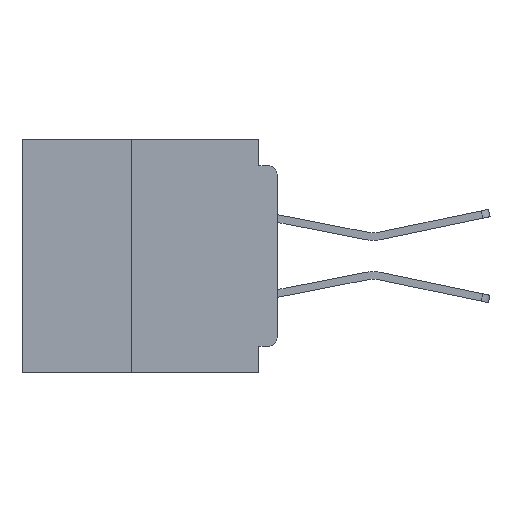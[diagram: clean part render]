
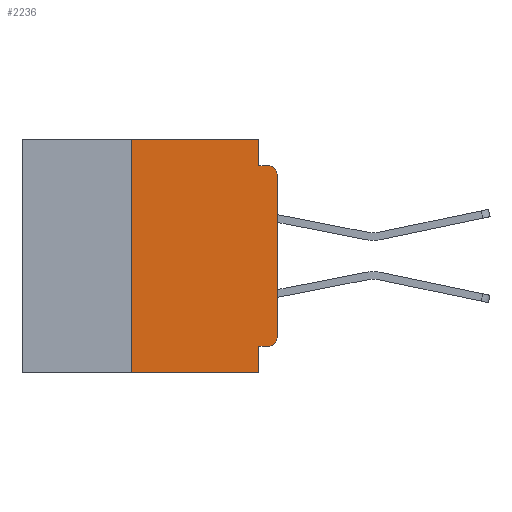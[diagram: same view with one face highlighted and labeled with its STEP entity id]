
A CAD part, left-side view. The second image highlights one B-rep face of the part: STEP entity #2236.
In plain terms, the highlighted planar face has unit normal (-1, 0, 0).
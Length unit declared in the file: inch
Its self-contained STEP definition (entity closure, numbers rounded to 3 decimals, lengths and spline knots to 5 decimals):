
#697 = CARTESIAN_POINT ( 'NONE',  ( 0., 0.031, -0.045 ) ) ;
#748 = CARTESIAN_POINT ( 'NONE',  ( 0., 0., -0.06 ) ) ;
#896 = CARTESIAN_POINT ( 'NONE',  ( 0., 0.031, -0.4 ) ) ;
#1283 = CARTESIAN_POINT ( 'NONE',  ( 0., 0.25, -0.4 ) ) ;
#1347 = ORIENTED_EDGE ( 'NONE', *, *, #12987, .F. ) ;
#2236 = ADVANCED_FACE ( 'NONE', ( #42134 ), #5109, .F. ) ;
#2611 = VECTOR ( 'NONE', #17663, 39.37008 ) ;
#3041 = DIRECTION ( 'NONE',  ( 0., 0., 1. ) ) ;
#3204 = DIRECTION ( 'NONE',  ( -1., 0., 0. ) ) ;
#4115 = CARTESIAN_POINT ( 'NONE',  ( 0., 0.031, 0. ) ) ;
#4848 = CIRCLE ( 'NONE', #32400, 0.015 ) ;
#5109 = PLANE ( 'NONE',  #37269 ) ;
#5693 = LINE ( 'NONE', #39878, #39560 ) ;
#6392 = EDGE_CURVE ( 'NONE', #26781, #35134, #4848, .T. ) ;
#7335 = CARTESIAN_POINT ( 'NONE',  ( 0., 0.25, -0.4 ) ) ;
#7347 = DIRECTION ( 'NONE',  ( 0., 1., 0. ) ) ;
#7950 = VERTEX_POINT ( 'NONE', #30938 ) ;
#8720 = CARTESIAN_POINT ( 'NONE',  ( 0., 0.015, -0.355 ) ) ;
#9623 = LINE ( 'NONE', #13942, #18341 ) ;
#9832 = ORIENTED_EDGE ( 'NONE', *, *, #38285, .F. ) ;
#10707 = CARTESIAN_POINT ( 'NONE',  ( 0., 0., -0.34 ) ) ;
#10911 = LINE ( 'NONE', #1283, #2611 ) ;
#11263 = CARTESIAN_POINT ( 'NONE',  ( 0., 0.015, -0.045 ) ) ;
#12987 = EDGE_CURVE ( 'NONE', #13130, #35134, #41984, .T. ) ;
#13096 = ORIENTED_EDGE ( 'NONE', *, *, #6392, .T. ) ;
#13130 = VERTEX_POINT ( 'NONE', #697 ) ;
#13190 = VERTEX_POINT ( 'NONE', #4115 ) ;
#13942 = CARTESIAN_POINT ( 'NONE',  ( 0., 0.031, 0. ) ) ;
#14481 = LINE ( 'NONE', #40150, #31872 ) ;
#14923 = EDGE_CURVE ( 'NONE', #35667, #20470, #40693, .T. ) ;
#15073 = DIRECTION ( 'NONE',  ( 1., 0., 0. ) ) ;
#15202 = ORIENTED_EDGE ( 'NONE', *, *, #20283, .T. ) ;
#15714 = VERTEX_POINT ( 'NONE', #10707 ) ;
#16179 = CARTESIAN_POINT ( 'NONE',  ( 0., 0.015, -0.06 ) ) ;
#16199 = VECTOR ( 'NONE', #3041, 39.37008 ) ;
#17250 = DIRECTION ( 'NONE',  ( 0., 0., -1. ) ) ;
#17405 = ORIENTED_EDGE ( 'NONE', *, *, #37001, .F. ) ;
#17663 = DIRECTION ( 'NONE',  ( 0., 0., 1. ) ) ;
#17851 = CIRCLE ( 'NONE', #31909, 0.015 ) ;
#17927 = VECTOR ( 'NONE', #25665, 39.37008 ) ;
#18206 = ORIENTED_EDGE ( 'NONE', *, *, #38445, .F. ) ;
#18341 = VECTOR ( 'NONE', #36856, 39.37008 ) ;
#19436 = EDGE_LOOP ( 'NONE', ( #21223, #13096, #1347, #17405, #40058, #18206, #31704, #24213, #9832, #15202 ) ) ;
#19444 = DIRECTION ( 'NONE',  ( 0., 0., -1. ) ) ;
#20283 = EDGE_CURVE ( 'NONE', #34707, #15714, #17851, .T. ) ;
#20470 = VERTEX_POINT ( 'NONE', #896 ) ;
#21223 = ORIENTED_EDGE ( 'NONE', *, *, #29830, .T. ) ;
#22875 = CARTESIAN_POINT ( 'NONE',  ( 0., 0.015, -0.34 ) ) ;
#22942 = DIRECTION ( 'NONE',  ( 0., -1., 0. ) ) ;
#23126 = VECTOR ( 'NONE', #32694, 39.37008 ) ;
#24213 = ORIENTED_EDGE ( 'NONE', *, *, #38310, .F. ) ;
#25665 = DIRECTION ( 'NONE',  ( 0., -1., 0. ) ) ;
#26162 = DIRECTION ( 'NONE',  ( 0., 0., -1. ) ) ;
#26227 = CARTESIAN_POINT ( 'NONE',  ( 0., 0.437, -0.4 ) ) ;
#26781 = VERTEX_POINT ( 'NONE', #748 ) ;
#29830 = EDGE_CURVE ( 'NONE', #15714, #26781, #33601, .T. ) ;
#30938 = CARTESIAN_POINT ( 'NONE',  ( 0., 0.031, -0.355 ) ) ;
#31704 = ORIENTED_EDGE ( 'NONE', *, *, #14923, .T. ) ;
#31846 = LINE ( 'NONE', #39163, #23126 ) ;
#31872 = VECTOR ( 'NONE', #17250, 39.37008 ) ;
#31909 = AXIS2_PLACEMENT_3D ( 'NONE', #22875, #3204, #26162 ) ;
#32002 = VECTOR ( 'NONE', #22942, 39.37008 ) ;
#32400 = AXIS2_PLACEMENT_3D ( 'NONE', #16179, #39080, #19444 ) ;
#32694 = DIRECTION ( 'NONE',  ( 0., -1., 0. ) ) ;
#33601 = LINE ( 'NONE', #39192, #16199 ) ;
#34665 = CARTESIAN_POINT ( 'NONE',  ( 0., 0.437, 0. ) ) ;
#34707 = VERTEX_POINT ( 'NONE', #8720 ) ;
#35134 = VERTEX_POINT ( 'NONE', #11263 ) ;
#35425 = CARTESIAN_POINT ( 'NONE',  ( 0., 0., -0.045 ) ) ;
#35667 = VERTEX_POINT ( 'NONE', #7335 ) ;
#36856 = DIRECTION ( 'NONE',  ( 0., 0., -1. ) ) ;
#37001 = EDGE_CURVE ( 'NONE', #13190, #13130, #9623, .T. ) ;
#37269 = AXIS2_PLACEMENT_3D ( 'NONE', #34665, #15073, #37981 ) ;
#37981 = DIRECTION ( 'NONE',  ( 0., 0., -1. ) ) ;
#38285 = EDGE_CURVE ( 'NONE', #34707, #7950, #5693, .T. ) ;
#38310 = EDGE_CURVE ( 'NONE', #7950, #20470, #14481, .T. ) ;
#38445 = EDGE_CURVE ( 'NONE', #35667, #42186, #10911, .T. ) ;
#39080 = DIRECTION ( 'NONE',  ( -1., 0., 0. ) ) ;
#39099 = CARTESIAN_POINT ( 'NONE',  ( 0., 0.25, 0. ) ) ;
#39163 = CARTESIAN_POINT ( 'NONE',  ( 0., 0.437, 0. ) ) ;
#39192 = CARTESIAN_POINT ( 'NONE',  ( 0., 0., 0. ) ) ;
#39437 = EDGE_CURVE ( 'NONE', #42186, #13190, #31846, .T. ) ;
#39560 = VECTOR ( 'NONE', #7347, 39.37008 ) ;
#39878 = CARTESIAN_POINT ( 'NONE',  ( 0., 0., -0.355 ) ) ;
#40058 = ORIENTED_EDGE ( 'NONE', *, *, #39437, .F. ) ;
#40150 = CARTESIAN_POINT ( 'NONE',  ( 0., 0.031, -0.4 ) ) ;
#40693 = LINE ( 'NONE', #26227, #32002 ) ;
#41984 = LINE ( 'NONE', #35425, #17927 ) ;
#42134 = FACE_OUTER_BOUND ( 'NONE', #19436, .T. ) ;
#42186 = VERTEX_POINT ( 'NONE', #39099 ) ;
